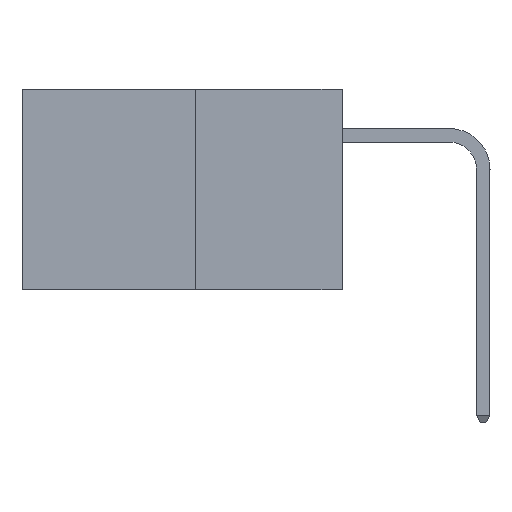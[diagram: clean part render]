
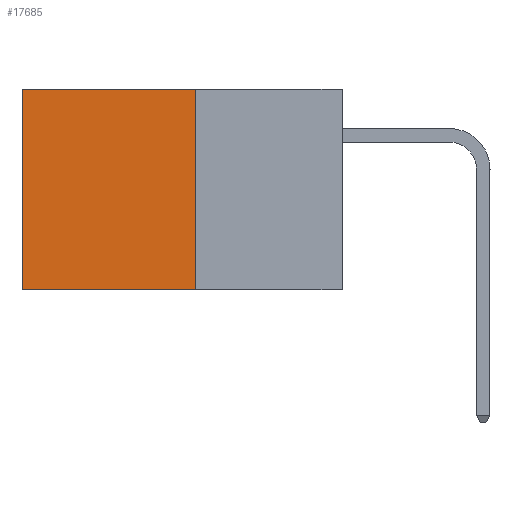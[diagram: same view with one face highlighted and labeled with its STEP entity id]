
A CAD part, left-side view. The second image highlights one B-rep face of the part: STEP entity #17685.
In plain terms, the highlighted planar face has unit normal (-1, 0, 0).
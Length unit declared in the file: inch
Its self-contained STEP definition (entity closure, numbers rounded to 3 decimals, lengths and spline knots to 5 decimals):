
#126 = VECTOR ( 'NONE', #5026, 39.37008 ) ;
#591 = VECTOR ( 'NONE', #8028, 39.37008 ) ;
#843 = CARTESIAN_POINT ( 'NONE',  ( 0.277, 0.27, -0.37 ) ) ;
#2070 = VERTEX_POINT ( 'NONE', #22837 ) ;
#5026 = DIRECTION ( 'NONE',  ( 0., 1., 0. ) ) ;
#5734 = DIRECTION ( 'NONE',  ( 1., 0., 0. ) ) ;
#5985 = CARTESIAN_POINT ( 'NONE',  ( 0.277, 0.59, -0.37 ) ) ;
#6418 = EDGE_CURVE ( 'NONE', #22044, #7294, #17954, .T. ) ;
#6851 = VECTOR ( 'NONE', #22419, 39.37008 ) ;
#7201 = ORIENTED_EDGE ( 'NONE', *, *, #19456, .T. ) ;
#7294 = VERTEX_POINT ( 'NONE', #12441 ) ;
#8028 = DIRECTION ( 'NONE',  ( 0., 0., -1. ) ) ;
#8574 = FACE_OUTER_BOUND ( 'NONE', #12746, .T. ) ;
#9159 = LINE ( 'NONE', #13539, #14084 ) ;
#11598 = LINE ( 'NONE', #5985, #591 ) ;
#12441 = CARTESIAN_POINT ( 'NONE',  ( 0.277, 0.27, -0.37 ) ) ;
#12746 = EDGE_LOOP ( 'NONE', ( #17585, #23836, #13426, #7201 ) ) ;
#13426 = ORIENTED_EDGE ( 'NONE', *, *, #6418, .F. ) ;
#13539 = CARTESIAN_POINT ( 'NONE',  ( 0.277, 0.27, 0. ) ) ;
#14084 = VECTOR ( 'NONE', #25718, 39.37008 ) ;
#15177 = CARTESIAN_POINT ( 'NONE',  ( 0.277, 0.27, 0. ) ) ;
#16710 = LINE ( 'NONE', #843, #126 ) ;
#17376 = VERTEX_POINT ( 'NONE', #21222 ) ;
#17585 = ORIENTED_EDGE ( 'NONE', *, *, #26285, .T. ) ;
#17685 = ADVANCED_FACE ( 'NONE', ( #8574 ), #26141, .F. ) ;
#17954 = LINE ( 'NONE', #22629, #6851 ) ;
#18186 = CARTESIAN_POINT ( 'NONE',  ( 0.277, 0.27, -0.37 ) ) ;
#19387 = EDGE_CURVE ( 'NONE', #7294, #2070, #16710, .T. ) ;
#19456 = EDGE_CURVE ( 'NONE', #22044, #17376, #9159, .T. ) ;
#20227 = DIRECTION ( 'NONE',  ( 0., 0., -1. ) ) ;
#21222 = CARTESIAN_POINT ( 'NONE',  ( 0.277, 0.59, 0. ) ) ;
#22044 = VERTEX_POINT ( 'NONE', #15177 ) ;
#22419 = DIRECTION ( 'NONE',  ( 0., 0., -1. ) ) ;
#22629 = CARTESIAN_POINT ( 'NONE',  ( 0.277, 0.27, -0.37 ) ) ;
#22837 = CARTESIAN_POINT ( 'NONE',  ( 0.277, 0.59, -0.37 ) ) ;
#23836 = ORIENTED_EDGE ( 'NONE', *, *, #19387, .F. ) ;
#24628 = AXIS2_PLACEMENT_3D ( 'NONE', #18186, #5734, #20227 ) ;
#25718 = DIRECTION ( 'NONE',  ( 0., 1., 0. ) ) ;
#26141 = PLANE ( 'NONE',  #24628 ) ;
#26285 = EDGE_CURVE ( 'NONE', #17376, #2070, #11598, .T. ) ;
